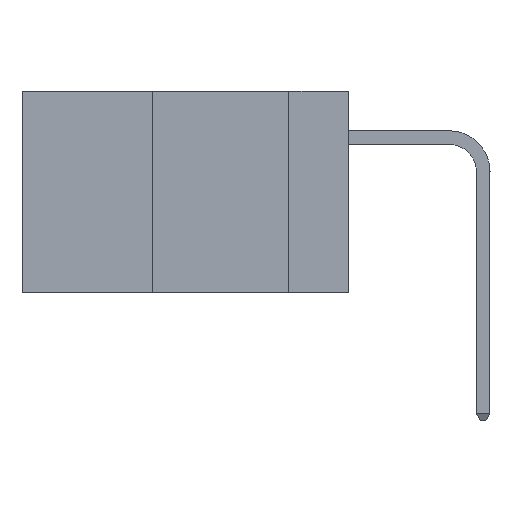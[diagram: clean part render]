
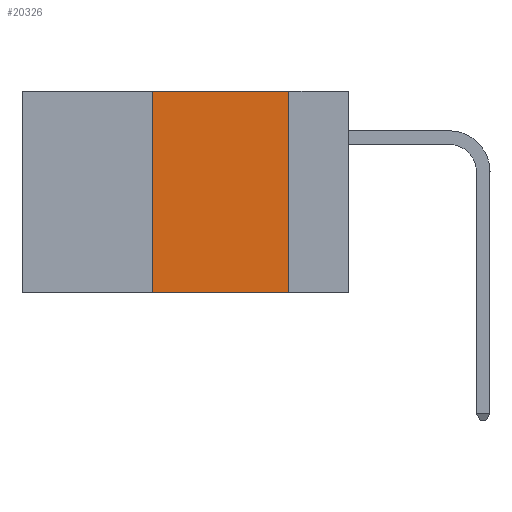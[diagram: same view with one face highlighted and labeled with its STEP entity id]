
A CAD part, left-side view. The second image highlights one B-rep face of the part: STEP entity #20326.
In plain terms, the highlighted planar face has unit normal (-1, 0, 0).
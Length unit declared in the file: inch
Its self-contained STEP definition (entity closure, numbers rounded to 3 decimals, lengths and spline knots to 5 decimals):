
#37 = CARTESIAN_POINT ( 'NONE',  ( 0., 0.6, 0. ) ) ;
#979 = EDGE_CURVE ( 'NONE', #31779, #28898, #10514, .T. ) ;
#3932 = VECTOR ( 'NONE', #30087, 39.37008 ) ;
#4795 = VECTOR ( 'NONE', #12061, 39.37008 ) ;
#5999 = VERTEX_POINT ( 'NONE', #7659 ) ;
#6994 = CARTESIAN_POINT ( 'NONE',  ( 0., 0.6, 0. ) ) ;
#7117 = CARTESIAN_POINT ( 'NONE',  ( 0., 0.36, 0. ) ) ;
#7338 = VECTOR ( 'NONE', #26900, 39.37008 ) ;
#7567 = EDGE_LOOP ( 'NONE', ( #18793, #16424, #14700, #24305 ) ) ;
#7659 = CARTESIAN_POINT ( 'NONE',  ( 0., 0.11, 0. ) ) ;
#8123 = LINE ( 'NONE', #37, #7338 ) ;
#8678 = EDGE_CURVE ( 'NONE', #31525, #5999, #8123, .T. ) ;
#9493 = PLANE ( 'NONE',  #21276 ) ;
#9777 = FACE_OUTER_BOUND ( 'NONE', #7567, .T. ) ;
#10310 = VECTOR ( 'NONE', #21811, 39.37008 ) ;
#10514 = LINE ( 'NONE', #25778, #3932 ) ;
#10918 = EDGE_CURVE ( 'NONE', #31779, #31525, #29836, .T. ) ;
#11281 = CARTESIAN_POINT ( 'NONE',  ( 0., 0.36, -0.37 ) ) ;
#11975 = DIRECTION ( 'NONE',  ( 0., 0., -1. ) ) ;
#12061 = DIRECTION ( 'NONE',  ( 0., 0., -1. ) ) ;
#14348 = DIRECTION ( 'NONE',  ( 1., 0., 0. ) ) ;
#14700 = ORIENTED_EDGE ( 'NONE', *, *, #10918, .F. ) ;
#15063 = CARTESIAN_POINT ( 'NONE',  ( 0., 0.11, -0.37 ) ) ;
#16424 = ORIENTED_EDGE ( 'NONE', *, *, #8678, .F. ) ;
#17926 = LINE ( 'NONE', #21775, #4795 ) ;
#18793 = ORIENTED_EDGE ( 'NONE', *, *, #30598, .F. ) ;
#20275 = CARTESIAN_POINT ( 'NONE',  ( 0., 0.36, 0. ) ) ;
#20326 = ADVANCED_FACE ( 'NONE', ( #9777 ), #9493, .F. ) ;
#21276 = AXIS2_PLACEMENT_3D ( 'NONE', #6994, #14348, #11975 ) ;
#21775 = CARTESIAN_POINT ( 'NONE',  ( 0., 0.11, 0. ) ) ;
#21811 = DIRECTION ( 'NONE',  ( 0., 0., 1. ) ) ;
#24305 = ORIENTED_EDGE ( 'NONE', *, *, #979, .T. ) ;
#25778 = CARTESIAN_POINT ( 'NONE',  ( 0., 0.6, -0.37 ) ) ;
#26900 = DIRECTION ( 'NONE',  ( 0., -1., 0. ) ) ;
#28898 = VERTEX_POINT ( 'NONE', #15063 ) ;
#29836 = LINE ( 'NONE', #7117, #10310 ) ;
#30087 = DIRECTION ( 'NONE',  ( 0., -1., 0. ) ) ;
#30598 = EDGE_CURVE ( 'NONE', #5999, #28898, #17926, .T. ) ;
#31525 = VERTEX_POINT ( 'NONE', #20275 ) ;
#31779 = VERTEX_POINT ( 'NONE', #11281 ) ;
